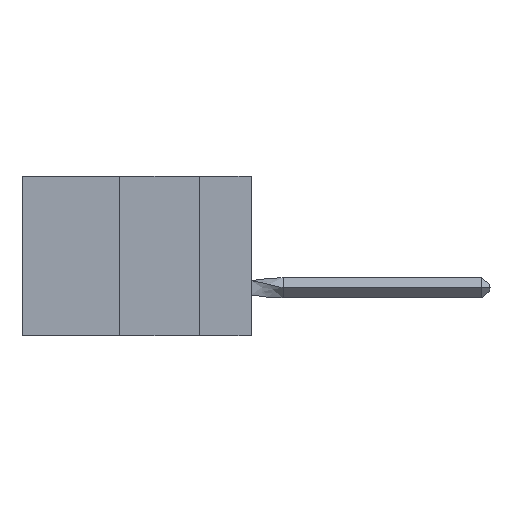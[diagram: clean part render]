
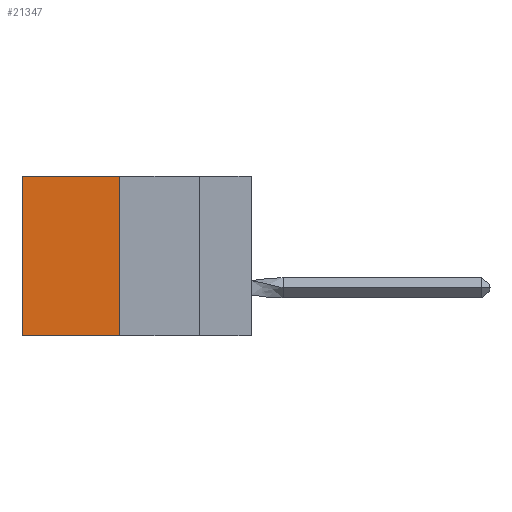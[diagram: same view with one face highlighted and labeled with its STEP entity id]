
A CAD part, left-side view. The second image highlights one B-rep face of the part: STEP entity #21347.
In plain terms, the highlighted planar face has unit normal (-1, 0, 0).
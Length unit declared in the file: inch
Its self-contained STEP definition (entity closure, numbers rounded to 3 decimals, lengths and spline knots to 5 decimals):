
#2332 = VECTOR ( 'NONE', #13329, 39.37008 ) ;
#2355 = VECTOR ( 'NONE', #12577, 39.37008 ) ;
#4240 = CARTESIAN_POINT ( 'NONE',  ( 0.305, 0.72, -0.5 ) ) ;
#7004 = VECTOR ( 'NONE', #16219, 39.37008 ) ;
#7390 = EDGE_CURVE ( 'NONE', #18878, #7784, #7527, .T. ) ;
#7527 = LINE ( 'NONE', #16411, #2355 ) ;
#7657 = EDGE_CURVE ( 'NONE', #18878, #10619, #21484, .T. ) ;
#7784 = VERTEX_POINT ( 'NONE', #18212 ) ;
#7867 = ORIENTED_EDGE ( 'NONE', *, *, #13506, .T. ) ;
#8181 = FACE_OUTER_BOUND ( 'NONE', #10655, .T. ) ;
#10619 = VERTEX_POINT ( 'NONE', #11810 ) ;
#10655 = EDGE_LOOP ( 'NONE', ( #7867, #12141, #16082, #17719 ) ) ;
#11504 = DIRECTION ( 'NONE',  ( 0., 1., 0. ) ) ;
#11810 = CARTESIAN_POINT ( 'NONE',  ( 0.305, 0.413, -0.5 ) ) ;
#12141 = ORIENTED_EDGE ( 'NONE', *, *, #12931, .F. ) ;
#12577 = DIRECTION ( 'NONE',  ( 0., 1., 0. ) ) ;
#12931 = EDGE_CURVE ( 'NONE', #10619, #16371, #18497, .T. ) ;
#13081 = CARTESIAN_POINT ( 'NONE',  ( 0.305, 0.413, 0. ) ) ;
#13329 = DIRECTION ( 'NONE',  ( 0., 0., -1. ) ) ;
#13506 = EDGE_CURVE ( 'NONE', #7784, #16371, #24954, .T. ) ;
#16082 = ORIENTED_EDGE ( 'NONE', *, *, #7657, .F. ) ;
#16131 = CARTESIAN_POINT ( 'NONE',  ( 0.305, 0.72, -0.5 ) ) ;
#16219 = DIRECTION ( 'NONE',  ( 0., 0., -1. ) ) ;
#16371 = VERTEX_POINT ( 'NONE', #4240 ) ;
#16411 = CARTESIAN_POINT ( 'NONE',  ( 0.305, 0.413, 0. ) ) ;
#16711 = DIRECTION ( 'NONE',  ( 1., 0., 0. ) ) ;
#16756 = AXIS2_PLACEMENT_3D ( 'NONE', #22556, #16711, #24530 ) ;
#17719 = ORIENTED_EDGE ( 'NONE', *, *, #7390, .T. ) ;
#18212 = CARTESIAN_POINT ( 'NONE',  ( 0.305, 0.72, 0. ) ) ;
#18497 = LINE ( 'NONE', #25034, #19396 ) ;
#18878 = VERTEX_POINT ( 'NONE', #13081 ) ;
#19396 = VECTOR ( 'NONE', #11504, 39.37008 ) ;
#21347 = ADVANCED_FACE ( 'NONE', ( #8181 ), #24445, .F. ) ;
#21357 = CARTESIAN_POINT ( 'NONE',  ( 0.305, 0.413, -0.5 ) ) ;
#21484 = LINE ( 'NONE', #21357, #2332 ) ;
#22556 = CARTESIAN_POINT ( 'NONE',  ( 0.305, 0.413, -0.5 ) ) ;
#24445 = PLANE ( 'NONE',  #16756 ) ;
#24530 = DIRECTION ( 'NONE',  ( 0., 0., -1. ) ) ;
#24954 = LINE ( 'NONE', #16131, #7004 ) ;
#25034 = CARTESIAN_POINT ( 'NONE',  ( 0.305, 0.413, -0.5 ) ) ;
